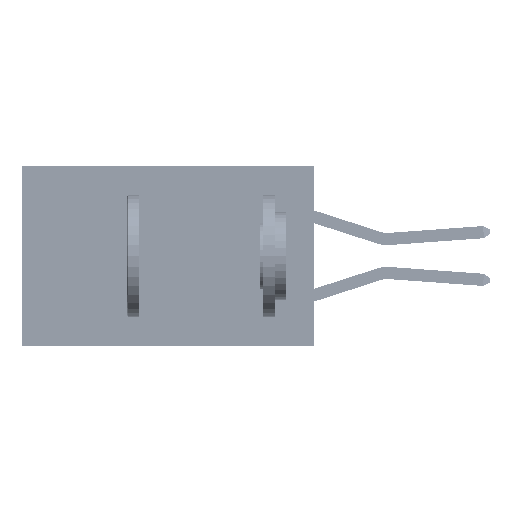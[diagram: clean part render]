
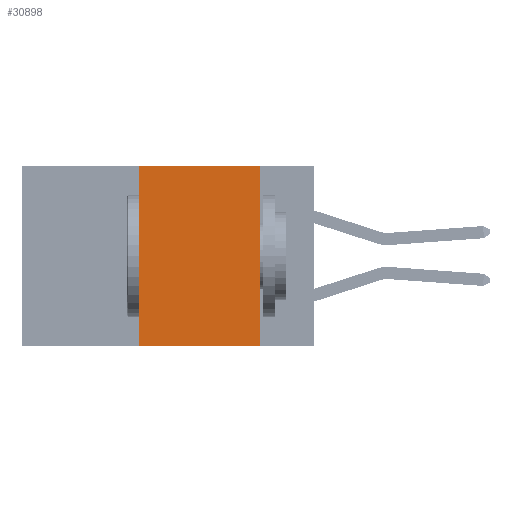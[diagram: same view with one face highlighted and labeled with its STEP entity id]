
A CAD part, left-side view. The second image highlights one B-rep face of the part: STEP entity #30898.
In plain terms, the highlighted planar face has unit normal (-1, 0, 0).
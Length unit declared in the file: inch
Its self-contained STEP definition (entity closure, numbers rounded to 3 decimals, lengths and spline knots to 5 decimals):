
#250 = EDGE_LOOP ( 'NONE', ( #21137, #28565, #10510, #26159 ) ) ;
#638 = DIRECTION ( 'NONE',  ( 1., 0., 0. ) ) ;
#1437 = VERTEX_POINT ( 'NONE', #42217 ) ;
#3422 = DIRECTION ( 'NONE',  ( 0., 0., -1. ) ) ;
#4251 = VECTOR ( 'NONE', #11243, 39.37008 ) ;
#5041 = PLANE ( 'NONE',  #50367 ) ;
#6721 = VECTOR ( 'NONE', #35313, 39.37008 ) ;
#6944 = LINE ( 'NONE', #39340, #47812 ) ;
#8206 = VECTOR ( 'NONE', #17177, 39.37008 ) ;
#8626 = LINE ( 'NONE', #35907, #4251 ) ;
#10491 = CARTESIAN_POINT ( 'NONE',  ( 0., 0.6, -0.37 ) ) ;
#10510 = ORIENTED_EDGE ( 'NONE', *, *, #26392, .F. ) ;
#11243 = DIRECTION ( 'NONE',  ( 0., 0., 1. ) ) ;
#12964 = DIRECTION ( 'NONE',  ( 0., 0., -1. ) ) ;
#14259 = CARTESIAN_POINT ( 'NONE',  ( 0., 0.36, -0.37 ) ) ;
#15387 = EDGE_CURVE ( 'NONE', #51431, #1437, #6944, .T. ) ;
#17177 = DIRECTION ( 'NONE',  ( 0., -1., 0. ) ) ;
#19094 = VERTEX_POINT ( 'NONE', #22452 ) ;
#21137 = ORIENTED_EDGE ( 'NONE', *, *, #15387, .F. ) ;
#21576 = CARTESIAN_POINT ( 'NONE',  ( 0., 0.6, 0. ) ) ;
#22452 = CARTESIAN_POINT ( 'NONE',  ( 0., 0.36, 0. ) ) ;
#26159 = ORIENTED_EDGE ( 'NONE', *, *, #29752, .T. ) ;
#26392 = EDGE_CURVE ( 'NONE', #27320, #19094, #8626, .T. ) ;
#27320 = VERTEX_POINT ( 'NONE', #14259 ) ;
#28565 = ORIENTED_EDGE ( 'NONE', *, *, #39379, .F. ) ;
#29752 = EDGE_CURVE ( 'NONE', #27320, #1437, #38915, .T. ) ;
#30898 = ADVANCED_FACE ( 'NONE', ( #47977 ), #5041, .F. ) ;
#33045 = CARTESIAN_POINT ( 'NONE',  ( 0., 0.6, 0. ) ) ;
#35313 = DIRECTION ( 'NONE',  ( 0., -1., 0. ) ) ;
#35907 = CARTESIAN_POINT ( 'NONE',  ( 0., 0.36, 0. ) ) ;
#38409 = CARTESIAN_POINT ( 'NONE',  ( 0., 0.11, 0. ) ) ;
#38915 = LINE ( 'NONE', #10491, #6721 ) ;
#39340 = CARTESIAN_POINT ( 'NONE',  ( 0., 0.11, 0. ) ) ;
#39379 = EDGE_CURVE ( 'NONE', #19094, #51431, #41609, .T. ) ;
#41609 = LINE ( 'NONE', #21576, #8206 ) ;
#42217 = CARTESIAN_POINT ( 'NONE',  ( 0., 0.11, -0.37 ) ) ;
#47812 = VECTOR ( 'NONE', #3422, 39.37008 ) ;
#47977 = FACE_OUTER_BOUND ( 'NONE', #250, .T. ) ;
#50367 = AXIS2_PLACEMENT_3D ( 'NONE', #33045, #638, #12964 ) ;
#51431 = VERTEX_POINT ( 'NONE', #38409 ) ;
